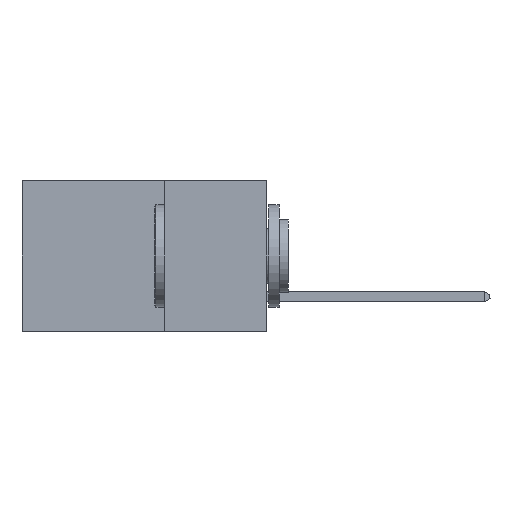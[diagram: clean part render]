
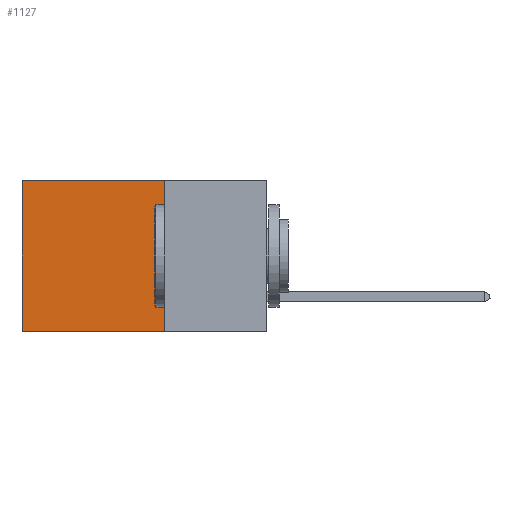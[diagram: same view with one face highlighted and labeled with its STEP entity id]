
A CAD part, left-side view. The second image highlights one B-rep face of the part: STEP entity #1127.
In plain terms, the highlighted planar face has unit normal (-1, 0, 0).
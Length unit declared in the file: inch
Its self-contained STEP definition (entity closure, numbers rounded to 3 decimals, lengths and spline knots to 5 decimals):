
#1127 = ADVANCED_FACE ( 'NONE', ( #14159 ), #29777, .F. ) ;
#2259 = ORIENTED_EDGE ( 'NONE', *, *, #26855, .F. ) ;
#2812 = LINE ( 'NONE', #25261, #8870 ) ;
#2983 = EDGE_CURVE ( 'NONE', #30820, #29735, #9640, .T. ) ;
#3398 = LINE ( 'NONE', #8898, #29027 ) ;
#3776 = LINE ( 'NONE', #28308, #32406 ) ;
#3862 = ORIENTED_EDGE ( 'NONE', *, *, #8784, .F. ) ;
#5449 = EDGE_LOOP ( 'NONE', ( #17037, #2259, #3862, #28092 ) ) ;
#5700 = VERTEX_POINT ( 'NONE', #24463 ) ;
#6709 = CARTESIAN_POINT ( 'NONE',  ( 0.2875, 0.6, -0.37 ) ) ;
#7700 = DIRECTION ( 'NONE',  ( 1., 0., 0. ) ) ;
#8784 = EDGE_CURVE ( 'NONE', #11823, #5700, #3398, .T. ) ;
#8870 = VECTOR ( 'NONE', #22707, 39.37008 ) ;
#8898 = CARTESIAN_POINT ( 'NONE',  ( 0.2875, 0.25, 0. ) ) ;
#9640 = LINE ( 'NONE', #10500, #22256 ) ;
#10500 = CARTESIAN_POINT ( 'NONE',  ( 0.2875, 0.6, 0. ) ) ;
#11823 = VERTEX_POINT ( 'NONE', #23300 ) ;
#14159 = FACE_OUTER_BOUND ( 'NONE', #5449, .T. ) ;
#14768 = AXIS2_PLACEMENT_3D ( 'NONE', #24367, #7700, #21664 ) ;
#17037 = ORIENTED_EDGE ( 'NONE', *, *, #2983, .T. ) ;
#21664 = DIRECTION ( 'NONE',  ( 0., 0., -1. ) ) ;
#22256 = VECTOR ( 'NONE', #29908, 39.37008 ) ;
#22707 = DIRECTION ( 'NONE',  ( 0., 1., 0. ) ) ;
#23300 = CARTESIAN_POINT ( 'NONE',  ( 0.2875, 0.25, 0. ) ) ;
#24367 = CARTESIAN_POINT ( 'NONE',  ( 0.2875, 0.25, 0. ) ) ;
#24463 = CARTESIAN_POINT ( 'NONE',  ( 0.2875, 0.25, -0.37 ) ) ;
#25261 = CARTESIAN_POINT ( 'NONE',  ( 0.2875, 0.25, 0. ) ) ;
#26855 = EDGE_CURVE ( 'NONE', #5700, #29735, #3776, .T. ) ;
#27493 = EDGE_CURVE ( 'NONE', #11823, #30820, #2812, .T. ) ;
#28092 = ORIENTED_EDGE ( 'NONE', *, *, #27493, .T. ) ;
#28308 = CARTESIAN_POINT ( 'NONE',  ( 0.2875, 0.25, -0.37 ) ) ;
#29027 = VECTOR ( 'NONE', #31089, 39.37008 ) ;
#29735 = VERTEX_POINT ( 'NONE', #6709 ) ;
#29777 = PLANE ( 'NONE',  #14768 ) ;
#29908 = DIRECTION ( 'NONE',  ( 0., 0., -1. ) ) ;
#30820 = VERTEX_POINT ( 'NONE', #31612 ) ;
#31081 = DIRECTION ( 'NONE',  ( 0., 1., 0. ) ) ;
#31089 = DIRECTION ( 'NONE',  ( 0., 0., -1. ) ) ;
#31612 = CARTESIAN_POINT ( 'NONE',  ( 0.2875, 0.6, 0. ) ) ;
#32406 = VECTOR ( 'NONE', #31081, 39.37008 ) ;
